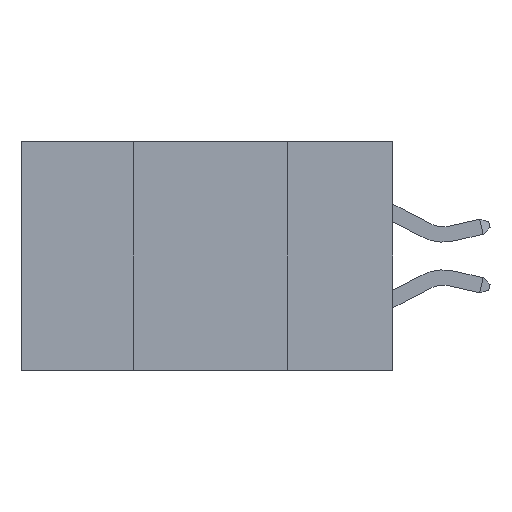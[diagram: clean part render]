
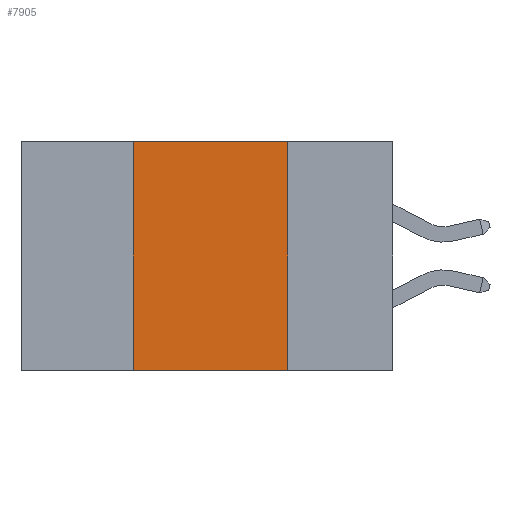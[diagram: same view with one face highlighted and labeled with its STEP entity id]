
A CAD part, left-side view. The second image highlights one B-rep face of the part: STEP entity #7905.
In plain terms, the highlighted planar face has unit normal (-1, 0, 0).
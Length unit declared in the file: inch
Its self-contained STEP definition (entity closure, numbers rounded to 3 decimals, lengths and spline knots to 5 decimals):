
#1074 = LINE ( 'NONE', #4398, #10751 ) ;
#2274 = VECTOR ( 'NONE', #8706, 39.37008 ) ;
#4398 = CARTESIAN_POINT ( 'NONE',  ( 0., 0.42, 0. ) ) ;
#5565 = LINE ( 'NONE', #23629, #9985 ) ;
#5720 = CARTESIAN_POINT ( 'NONE',  ( 0., 0.6, 0. ) ) ;
#6817 = CARTESIAN_POINT ( 'NONE',  ( 0., 0.17, 0. ) ) ;
#6977 = LINE ( 'NONE', #16663, #16320 ) ;
#7089 = CARTESIAN_POINT ( 'NONE',  ( 0., 0.17, 0. ) ) ;
#7378 = DIRECTION ( 'NONE',  ( 0., -1., 0. ) ) ;
#7496 = VERTEX_POINT ( 'NONE', #17595 ) ;
#7604 = EDGE_CURVE ( 'NONE', #17454, #16842, #8094, .T. ) ;
#7652 = PLANE ( 'NONE',  #21626 ) ;
#7781 = ORIENTED_EDGE ( 'NONE', *, *, #14941, .T. ) ;
#7905 = ADVANCED_FACE ( 'NONE', ( #10406 ), #7652, .F. ) ;
#8092 = CARTESIAN_POINT ( 'NONE',  ( 0., 0.42, 0. ) ) ;
#8094 = LINE ( 'NONE', #6817, #2274 ) ;
#8706 = DIRECTION ( 'NONE',  ( 0., 0., -1. ) ) ;
#9512 = DIRECTION ( 'NONE',  ( 1., 0., 0. ) ) ;
#9985 = VECTOR ( 'NONE', #21876, 39.37008 ) ;
#10406 = FACE_OUTER_BOUND ( 'NONE', #17862, .T. ) ;
#10418 = EDGE_CURVE ( 'NONE', #10677, #17454, #6977, .T. ) ;
#10677 = VERTEX_POINT ( 'NONE', #8092 ) ;
#10751 = VECTOR ( 'NONE', #19370, 39.37008 ) ;
#13720 = ORIENTED_EDGE ( 'NONE', *, *, #7604, .F. ) ;
#14941 = EDGE_CURVE ( 'NONE', #7496, #16842, #5565, .T. ) ;
#16320 = VECTOR ( 'NONE', #7378, 39.37008 ) ;
#16663 = CARTESIAN_POINT ( 'NONE',  ( 0., 0.6, 0. ) ) ;
#16842 = VERTEX_POINT ( 'NONE', #18403 ) ;
#17454 = VERTEX_POINT ( 'NONE', #7089 ) ;
#17595 = CARTESIAN_POINT ( 'NONE',  ( 0., 0.42, -0.37 ) ) ;
#17862 = EDGE_LOOP ( 'NONE', ( #13720, #19020, #18253, #7781 ) ) ;
#18253 = ORIENTED_EDGE ( 'NONE', *, *, #20716, .F. ) ;
#18403 = CARTESIAN_POINT ( 'NONE',  ( 0., 0.17, -0.37 ) ) ;
#19020 = ORIENTED_EDGE ( 'NONE', *, *, #10418, .F. ) ;
#19370 = DIRECTION ( 'NONE',  ( 0., 0., 1. ) ) ;
#20716 = EDGE_CURVE ( 'NONE', #7496, #10677, #1074, .T. ) ;
#21626 = AXIS2_PLACEMENT_3D ( 'NONE', #5720, #9512, #22312 ) ;
#21876 = DIRECTION ( 'NONE',  ( 0., -1., 0. ) ) ;
#22312 = DIRECTION ( 'NONE',  ( 0., 0., -1. ) ) ;
#23629 = CARTESIAN_POINT ( 'NONE',  ( 0., 0.6, -0.37 ) ) ;
